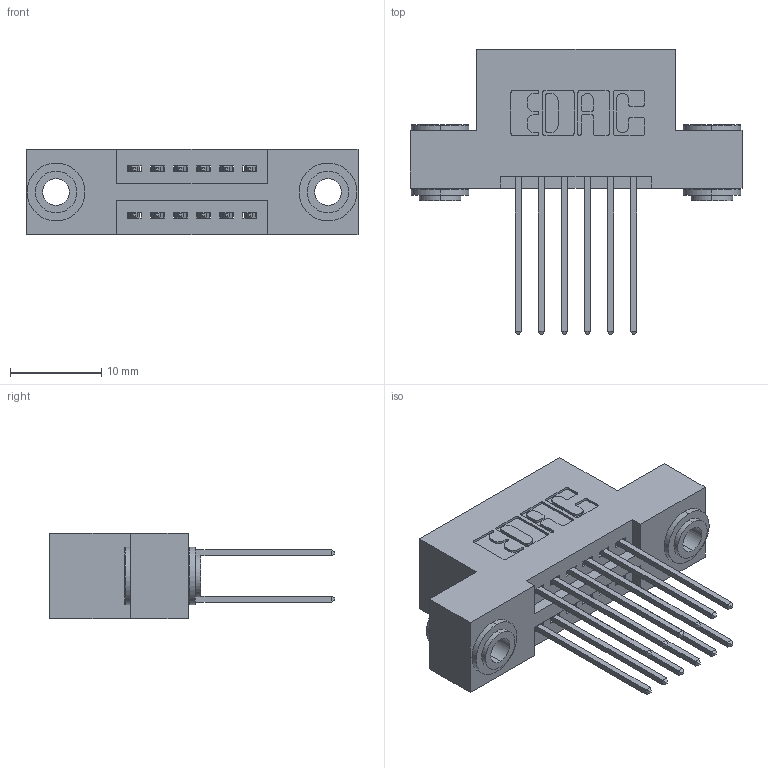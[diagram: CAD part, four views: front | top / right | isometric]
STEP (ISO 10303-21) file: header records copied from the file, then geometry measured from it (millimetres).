
FILE_DESCRIPTION (( 'STEP AP203' ), '1' );
FILE_NAME ('395-012-542-203.STEP', '2018-11-05T18:14:32', ( '' ), ( '' ), 'SwSTEP 2.0', 'SolidWorks 2016', '' );
FILE_SCHEMA (( 'CONFIG_CONTROL_DESIGN' ));
Length unit declared in the file: inch
Products named in the file (4): 345-250-002_345-250-002-102; 345-292-001_345-293-142; 345 Part_Flush Mounting Lugs - 0.156 Dia-TH; 395-012-542-203
Assembly tree (15 placements, depth 2):
  395-012-542-203
    345 Part_Flush Mounting Lugs - 0.156 Dia-TH
    345-292-001_345-293-142  x12
    345-250-002_345-250-002-102  x2
Bounding box: 36.45 x 31.29 x 9.4 mm (x, y, z)
Volume: 3281.9 mm3; surface area: 4620.2 mm2
Topology: 15 solids, 15 shells, 764 faces, 2205 edges, 1450 vertices
Faces by surface type: plane 486, cylinder 270, cone 8
Entity records: 10222 total; most frequent: CARTESIAN_POINT 1723, ORIENTED_EDGE 1650, DIRECTION 1595, EDGE_CURVE 825, VECTOR 645, LINE 645, VERTEX_POINT 546, AXIS2_PLACEMENT_3D 475
